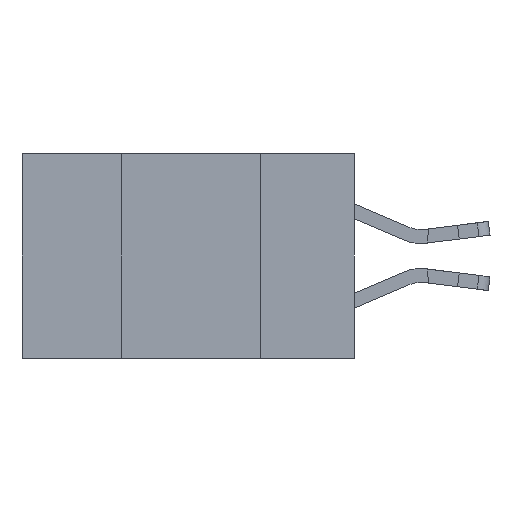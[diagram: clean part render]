
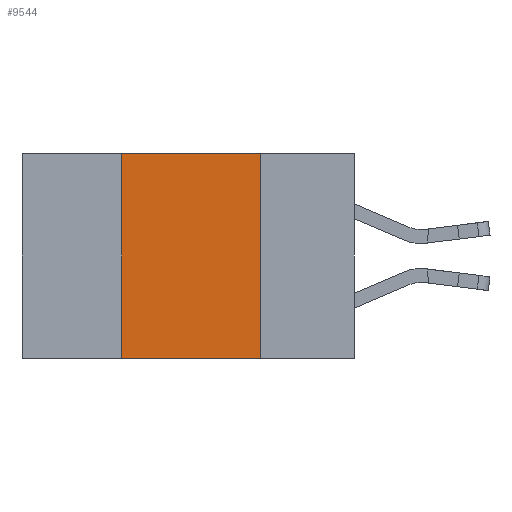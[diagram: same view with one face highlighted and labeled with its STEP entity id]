
A CAD part, left-side view. The second image highlights one B-rep face of the part: STEP entity #9544.
In plain terms, the highlighted planar face has unit normal (-1, 0, 0).
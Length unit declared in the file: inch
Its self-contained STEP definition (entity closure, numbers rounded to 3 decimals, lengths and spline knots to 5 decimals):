
#42 = CARTESIAN_POINT ( 'NONE',  ( 0., 0.6, 0. ) ) ;
#109 = CARTESIAN_POINT ( 'NONE',  ( 0., 0.42, -0.37 ) ) ;
#238 = VERTEX_POINT ( 'NONE', #4034 ) ;
#739 = EDGE_CURVE ( 'NONE', #7246, #238, #8027, .T. ) ;
#1304 = ORIENTED_EDGE ( 'NONE', *, *, #739, .F. ) ;
#1979 = VECTOR ( 'NONE', #15284, 39.37008 ) ;
#2194 = LINE ( 'NONE', #9003, #1979 ) ;
#2864 = DIRECTION ( 'NONE',  ( 0., -1., 0. ) ) ;
#3993 = VERTEX_POINT ( 'NONE', #109 ) ;
#4034 = CARTESIAN_POINT ( 'NONE',  ( 0., 0.17, -0.37 ) ) ;
#4174 = CARTESIAN_POINT ( 'NONE',  ( 0., 0.17, -0.37 ) ) ;
#4836 = CARTESIAN_POINT ( 'NONE',  ( 0., 0.42, 0. ) ) ;
#5065 = ORIENTED_EDGE ( 'NONE', *, *, #10658, .T. ) ;
#5153 = DIRECTION ( 'NONE',  ( 0., -1., 0. ) ) ;
#5731 = CARTESIAN_POINT ( 'NONE',  ( 0., 0.6, -0.37 ) ) ;
#6128 = DIRECTION ( 'NONE',  ( 1., 0., 0. ) ) ;
#6137 = VERTEX_POINT ( 'NONE', #4836 ) ;
#6636 = DIRECTION ( 'NONE',  ( 0., 0., -1. ) ) ;
#7246 = VERTEX_POINT ( 'NONE', #7855 ) ;
#7612 = FACE_OUTER_BOUND ( 'NONE', #8417, .T. ) ;
#7702 = CARTESIAN_POINT ( 'NONE',  ( 0., 0.6, 0. ) ) ;
#7855 = CARTESIAN_POINT ( 'NONE',  ( 0., 0.17, 0. ) ) ;
#8027 = LINE ( 'NONE', #4174, #10230 ) ;
#8417 = EDGE_LOOP ( 'NONE', ( #1304, #12655, #13541, #5065 ) ) ;
#9003 = CARTESIAN_POINT ( 'NONE',  ( 0., 0.42, -0.37 ) ) ;
#9288 = VECTOR ( 'NONE', #2864, 39.37008 ) ;
#9544 = ADVANCED_FACE ( 'NONE', ( #7612 ), #16874, .F. ) ;
#9682 = LINE ( 'NONE', #5731, #9288 ) ;
#10230 = VECTOR ( 'NONE', #6636, 39.37008 ) ;
#10658 = EDGE_CURVE ( 'NONE', #3993, #238, #9682, .T. ) ;
#11634 = LINE ( 'NONE', #42, #12016 ) ;
#12016 = VECTOR ( 'NONE', #5153, 39.37008 ) ;
#12655 = ORIENTED_EDGE ( 'NONE', *, *, #13242, .F. ) ;
#12930 = DIRECTION ( 'NONE',  ( 0., 0., -1. ) ) ;
#13242 = EDGE_CURVE ( 'NONE', #6137, #7246, #11634, .T. ) ;
#13541 = ORIENTED_EDGE ( 'NONE', *, *, #15678, .F. ) ;
#13578 = AXIS2_PLACEMENT_3D ( 'NONE', #7702, #6128, #12930 ) ;
#15284 = DIRECTION ( 'NONE',  ( 0., 0., 1. ) ) ;
#15678 = EDGE_CURVE ( 'NONE', #3993, #6137, #2194, .T. ) ;
#16874 = PLANE ( 'NONE',  #13578 ) ;
